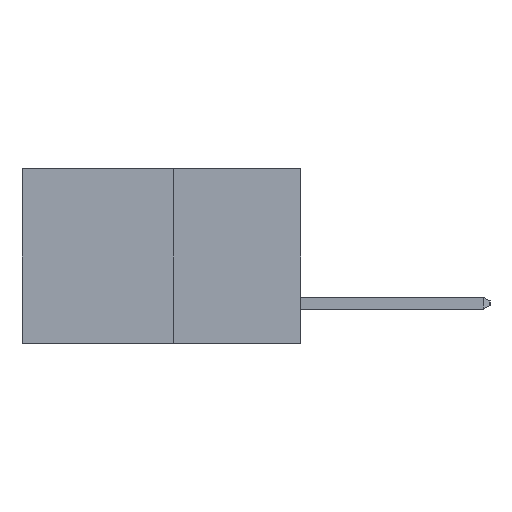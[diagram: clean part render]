
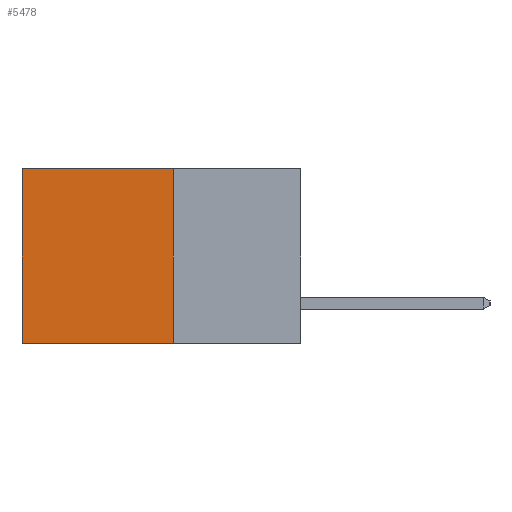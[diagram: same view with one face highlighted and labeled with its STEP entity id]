
A CAD part, left-side view. The second image highlights one B-rep face of the part: STEP entity #5478.
In plain terms, the highlighted planar face has unit normal (-1, 0, 0).
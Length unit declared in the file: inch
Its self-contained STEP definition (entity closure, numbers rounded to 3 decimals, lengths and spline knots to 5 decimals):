
#354 = VERTEX_POINT ( 'NONE', #6928 ) ;
#1249 = VECTOR ( 'NONE', #14666, 39.37008 ) ;
#1986 = ORIENTED_EDGE ( 'NONE', *, *, #13891, .F. ) ;
#3944 = EDGE_CURVE ( 'NONE', #354, #10859, #9840, .T. ) ;
#4534 = CARTESIAN_POINT ( 'NONE',  ( 0.277, 0.27, 0. ) ) ;
#4795 = LINE ( 'NONE', #4534, #16257 ) ;
#5478 = ADVANCED_FACE ( 'NONE', ( #12311 ), #15254, .F. ) ;
#5586 = ORIENTED_EDGE ( 'NONE', *, *, #11032, .F. ) ;
#6081 = DIRECTION ( 'NONE',  ( 0., 1., 0. ) ) ;
#6928 = CARTESIAN_POINT ( 'NONE',  ( 0.277, 0.59, 0. ) ) ;
#8134 = CARTESIAN_POINT ( 'NONE',  ( 0.277, 0.27, -0.37 ) ) ;
#9145 = ORIENTED_EDGE ( 'NONE', *, *, #3944, .T. ) ;
#9742 = VECTOR ( 'NONE', #14140, 39.37008 ) ;
#9840 = LINE ( 'NONE', #19096, #1249 ) ;
#10065 = ORIENTED_EDGE ( 'NONE', *, *, #13932, .T. ) ;
#10859 = VERTEX_POINT ( 'NONE', #11852 ) ;
#11032 = EDGE_CURVE ( 'NONE', #13261, #10859, #13712, .T. ) ;
#11645 = CARTESIAN_POINT ( 'NONE',  ( 0.277, 0.27, -0.37 ) ) ;
#11852 = CARTESIAN_POINT ( 'NONE',  ( 0.277, 0.59, -0.37 ) ) ;
#12073 = VERTEX_POINT ( 'NONE', #19369 ) ;
#12311 = FACE_OUTER_BOUND ( 'NONE', #15248, .T. ) ;
#12877 = DIRECTION ( 'NONE',  ( 0., 0., -1. ) ) ;
#13261 = VERTEX_POINT ( 'NONE', #11645 ) ;
#13712 = LINE ( 'NONE', #8134, #9742 ) ;
#13891 = EDGE_CURVE ( 'NONE', #12073, #13261, #17633, .T. ) ;
#13932 = EDGE_CURVE ( 'NONE', #12073, #354, #4795, .T. ) ;
#13998 = DIRECTION ( 'NONE',  ( 1., 0., 0. ) ) ;
#14140 = DIRECTION ( 'NONE',  ( 0., 1., 0. ) ) ;
#14201 = VECTOR ( 'NONE', #17851, 39.37008 ) ;
#14555 = CARTESIAN_POINT ( 'NONE',  ( 0.277, 0.27, -0.37 ) ) ;
#14666 = DIRECTION ( 'NONE',  ( 0., 0., -1. ) ) ;
#14902 = CARTESIAN_POINT ( 'NONE',  ( 0.277, 0.27, -0.37 ) ) ;
#15248 = EDGE_LOOP ( 'NONE', ( #9145, #5586, #1986, #10065 ) ) ;
#15254 = PLANE ( 'NONE',  #18122 ) ;
#16257 = VECTOR ( 'NONE', #6081, 39.37008 ) ;
#17633 = LINE ( 'NONE', #14902, #14201 ) ;
#17851 = DIRECTION ( 'NONE',  ( 0., 0., -1. ) ) ;
#18122 = AXIS2_PLACEMENT_3D ( 'NONE', #14555, #13998, #12877 ) ;
#19096 = CARTESIAN_POINT ( 'NONE',  ( 0.277, 0.59, -0.37 ) ) ;
#19369 = CARTESIAN_POINT ( 'NONE',  ( 0.277, 0.27, 0. ) ) ;
